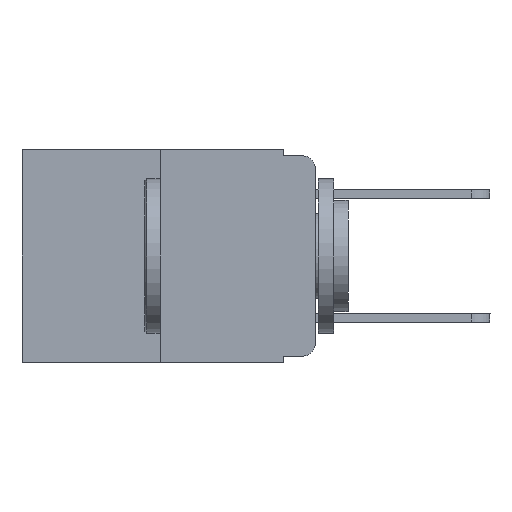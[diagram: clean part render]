
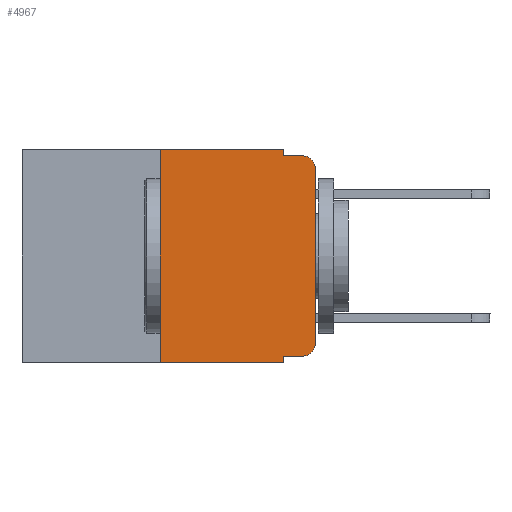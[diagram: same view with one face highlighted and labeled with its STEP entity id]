
A CAD part, left-side view. The second image highlights one B-rep face of the part: STEP entity #4967.
In plain terms, the highlighted planar face has unit normal (-1, 0, 0).
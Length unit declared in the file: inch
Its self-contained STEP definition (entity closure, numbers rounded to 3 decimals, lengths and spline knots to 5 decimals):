
#385 = DIRECTION ( 'NONE',  ( 0., 0., -1. ) ) ;
#425 = AXIS2_PLACEMENT_3D ( 'NONE', #14327, #23918, #23998 ) ;
#552 = CARTESIAN_POINT ( 'NONE',  ( 0., 0.051, -0.333 ) ) ;
#873 = DIRECTION ( 'NONE',  ( 0., -1., 0. ) ) ;
#914 = ORIENTED_EDGE ( 'NONE', *, *, #12873, .T. ) ;
#1680 = VECTOR ( 'NONE', #14603, 39.37008 ) ;
#1951 = VERTEX_POINT ( 'NONE', #5145 ) ;
#2330 = CARTESIAN_POINT ( 'NONE',  ( 0., 0.051, -0.01 ) ) ;
#2791 = EDGE_CURVE ( 'NONE', #10668, #3869, #19450, .T. ) ;
#2804 = CARTESIAN_POINT ( 'NONE',  ( 0., 0.051, -0.333 ) ) ;
#2898 = EDGE_LOOP ( 'NONE', ( #914, #14262, #18906, #20882, #13048, #20158, #10816, #5643, #22410, #18226 ) ) ;
#3452 = EDGE_CURVE ( 'NONE', #17037, #13411, #5783, .T. ) ;
#3673 = VERTEX_POINT ( 'NONE', #2804 ) ;
#3869 = VERTEX_POINT ( 'NONE', #2330 ) ;
#4041 = EDGE_CURVE ( 'NONE', #3673, #17966, #6320, .T. ) ;
#4490 = VERTEX_POINT ( 'NONE', #4977 ) ;
#4498 = VECTOR ( 'NONE', #12875, 39.37008 ) ;
#4569 = DIRECTION ( 'NONE',  ( 0., 0., -1. ) ) ;
#4822 = DIRECTION ( 'NONE',  ( 0., 0., -1. ) ) ;
#4967 = ADVANCED_FACE ( 'NONE', ( #15221 ), #22101, .F. ) ;
#4977 = CARTESIAN_POINT ( 'NONE',  ( 0., 0., -0.313 ) ) ;
#5145 = CARTESIAN_POINT ( 'NONE',  ( 0., 0.25, 0. ) ) ;
#5483 = VECTOR ( 'NONE', #385, 39.37008 ) ;
#5545 = LINE ( 'NONE', #16517, #1680 ) ;
#5643 = ORIENTED_EDGE ( 'NONE', *, *, #18170, .F. ) ;
#5783 = CIRCLE ( 'NONE', #16919, 0.02 ) ;
#6055 = VERTEX_POINT ( 'NONE', #19327 ) ;
#6198 = AXIS2_PLACEMENT_3D ( 'NONE', #16193, #6955, #4822 ) ;
#6320 = LINE ( 'NONE', #552, #24513 ) ;
#6452 = VECTOR ( 'NONE', #20702, 39.37008 ) ;
#6955 = DIRECTION ( 'NONE',  ( -1., 0., 0. ) ) ;
#7017 = EDGE_CURVE ( 'NONE', #20152, #6055, #18374, .T. ) ;
#7935 = VECTOR ( 'NONE', #11150, 39.37008 ) ;
#8301 = DIRECTION ( 'NONE',  ( -1., 0., 0. ) ) ;
#8609 = CARTESIAN_POINT ( 'NONE',  ( 0., 0.25, 0. ) ) ;
#8968 = CARTESIAN_POINT ( 'NONE',  ( 0., 0., 0. ) ) ;
#9994 = CARTESIAN_POINT ( 'NONE',  ( 0., 0.051, 0. ) ) ;
#10311 = VECTOR ( 'NONE', #21930, 39.37008 ) ;
#10668 = VERTEX_POINT ( 'NONE', #9994 ) ;
#10816 = ORIENTED_EDGE ( 'NONE', *, *, #7017, .T. ) ;
#11150 = DIRECTION ( 'NONE',  ( 0., 0., 1. ) ) ;
#11458 = EDGE_CURVE ( 'NONE', #17966, #4490, #20238, .T. ) ;
#11622 = DIRECTION ( 'NONE',  ( 0., -1., 0. ) ) ;
#11771 = CARTESIAN_POINT ( 'NONE',  ( 0., 0.02, -0.333 ) ) ;
#11980 = VECTOR ( 'NONE', #11622, 39.37008 ) ;
#12039 = CARTESIAN_POINT ( 'NONE',  ( 0., 0.02, -0.03 ) ) ;
#12447 = CARTESIAN_POINT ( 'NONE',  ( 0., 0., -0.03 ) ) ;
#12873 = EDGE_CURVE ( 'NONE', #4490, #17037, #17516, .T. ) ;
#12875 = DIRECTION ( 'NONE',  ( 0., -1., 0. ) ) ;
#13025 = CARTESIAN_POINT ( 'NONE',  ( 0., 0.25, -0.343 ) ) ;
#13048 = ORIENTED_EDGE ( 'NONE', *, *, #20118, .F. ) ;
#13398 = LINE ( 'NONE', #18857, #4498 ) ;
#13411 = VERTEX_POINT ( 'NONE', #17921 ) ;
#14262 = ORIENTED_EDGE ( 'NONE', *, *, #3452, .T. ) ;
#14327 = CARTESIAN_POINT ( 'NONE',  ( 0., 0.473, 0. ) ) ;
#14603 = DIRECTION ( 'NONE',  ( 0., 0., -1. ) ) ;
#15221 = FACE_OUTER_BOUND ( 'NONE', #2898, .T. ) ;
#15545 = LINE ( 'NONE', #16803, #11980 ) ;
#16193 = CARTESIAN_POINT ( 'NONE',  ( 0., 0.02, -0.313 ) ) ;
#16244 = LINE ( 'NONE', #8609, #10311 ) ;
#16517 = CARTESIAN_POINT ( 'NONE',  ( 0., 0.051, 0. ) ) ;
#16803 = CARTESIAN_POINT ( 'NONE',  ( 0., 0.051, -0.01 ) ) ;
#16875 = CARTESIAN_POINT ( 'NONE',  ( 0., 0.473, -0.343 ) ) ;
#16919 = AXIS2_PLACEMENT_3D ( 'NONE', #12039, #8301, #4569 ) ;
#17037 = VERTEX_POINT ( 'NONE', #12447 ) ;
#17516 = LINE ( 'NONE', #8968, #7935 ) ;
#17921 = CARTESIAN_POINT ( 'NONE',  ( 0., 0.02, -0.01 ) ) ;
#17966 = VERTEX_POINT ( 'NONE', #11771 ) ;
#18096 = EDGE_CURVE ( 'NONE', #20152, #1951, #16244, .T. ) ;
#18170 = EDGE_CURVE ( 'NONE', #3673, #6055, #5545, .T. ) ;
#18226 = ORIENTED_EDGE ( 'NONE', *, *, #11458, .T. ) ;
#18374 = LINE ( 'NONE', #16875, #6452 ) ;
#18857 = CARTESIAN_POINT ( 'NONE',  ( 0., 0.473, 0. ) ) ;
#18906 = ORIENTED_EDGE ( 'NONE', *, *, #22309, .F. ) ;
#19223 = CARTESIAN_POINT ( 'NONE',  ( 0., 0.051, 0. ) ) ;
#19327 = CARTESIAN_POINT ( 'NONE',  ( 0., 0.051, -0.343 ) ) ;
#19450 = LINE ( 'NONE', #19223, #5483 ) ;
#20118 = EDGE_CURVE ( 'NONE', #1951, #10668, #13398, .T. ) ;
#20152 = VERTEX_POINT ( 'NONE', #13025 ) ;
#20158 = ORIENTED_EDGE ( 'NONE', *, *, #18096, .F. ) ;
#20238 = CIRCLE ( 'NONE', #6198, 0.02 ) ;
#20702 = DIRECTION ( 'NONE',  ( 0., -1., 0. ) ) ;
#20882 = ORIENTED_EDGE ( 'NONE', *, *, #2791, .F. ) ;
#21930 = DIRECTION ( 'NONE',  ( 0., 0., 1. ) ) ;
#22101 = PLANE ( 'NONE',  #425 ) ;
#22309 = EDGE_CURVE ( 'NONE', #3869, #13411, #15545, .T. ) ;
#22410 = ORIENTED_EDGE ( 'NONE', *, *, #4041, .T. ) ;
#23918 = DIRECTION ( 'NONE',  ( 1., 0., 0. ) ) ;
#23998 = DIRECTION ( 'NONE',  ( 0., 0., -1. ) ) ;
#24513 = VECTOR ( 'NONE', #873, 39.37008 ) ;
